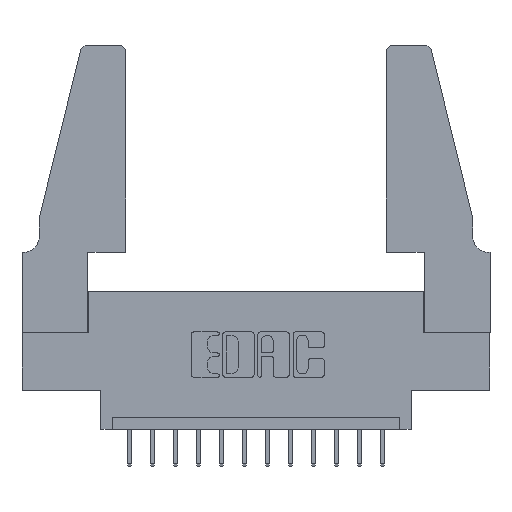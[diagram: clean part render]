
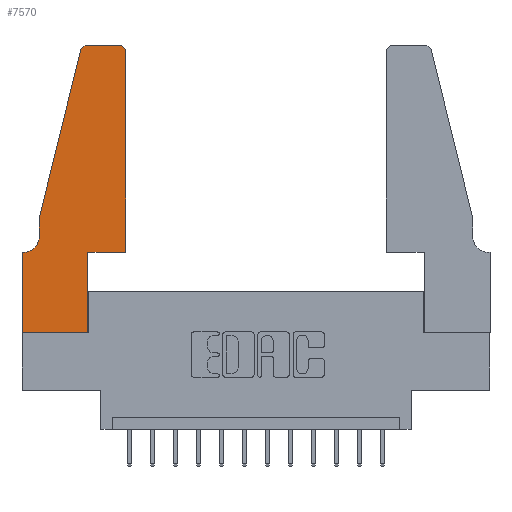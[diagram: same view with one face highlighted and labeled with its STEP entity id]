
A CAD part, top view. The second image highlights one B-rep face of the part: STEP entity #7570.
In plain terms, the highlighted planar face has unit normal (0, 0, 1).
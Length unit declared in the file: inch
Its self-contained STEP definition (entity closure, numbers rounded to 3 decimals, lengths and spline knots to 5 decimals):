
#68 = DIRECTION ( 'NONE',  ( 1., 0., 0. ) ) ;
#298 = CARTESIAN_POINT ( 'NONE',  ( 0.284, 1.22, 0.37 ) ) ;
#431 = VECTOR ( 'NONE', #9985, 39.37008 ) ;
#708 = EDGE_CURVE ( 'NONE', #6608, #3818, #10420, .T. ) ;
#802 = CIRCLE ( 'NONE', #4321, 0.03 ) ;
#808 = ORIENTED_EDGE ( 'NONE', *, *, #11677, .T. ) ;
#884 = DIRECTION ( 'NONE',  ( 0., 0., -1. ) ) ;
#943 = ORIENTED_EDGE ( 'NONE', *, *, #7886, .T. ) ;
#946 = CARTESIAN_POINT ( 'NONE',  ( 0.0755, 0.5, 0.37 ) ) ;
#1165 = ORIENTED_EDGE ( 'NONE', *, *, #3841, .T. ) ;
#1314 = CARTESIAN_POINT ( 'NONE',  ( 0.4205, 1.22, 0.37 ) ) ;
#1512 = DIRECTION ( 'NONE',  ( 0., 0., 1. ) ) ;
#1596 = CARTESIAN_POINT ( 'NONE',  ( 0., 0., 0.37 ) ) ;
#1765 = DIRECTION ( 'NONE',  ( -1., 0., 0. ) ) ;
#1864 = CARTESIAN_POINT ( 'NONE',  ( 0.4505, 1.22, 0.37 ) ) ;
#1882 = AXIS2_PLACEMENT_3D ( 'NONE', #9952, #1512, #10059 ) ;
#1934 = CARTESIAN_POINT ( 'NONE',  ( 0.0055, 0.35, 0.37 ) ) ;
#2064 = ORIENTED_EDGE ( 'NONE', *, *, #13709, .T. ) ;
#2082 = DIRECTION ( 'NONE',  ( -1., 0., 0. ) ) ;
#2103 = LINE ( 'NONE', #9622, #11247 ) ;
#2269 = CARTESIAN_POINT ( 'NONE',  ( 0.0755, 0.5, 0.37 ) ) ;
#2317 = DIRECTION ( 'NONE',  ( 0., 1., 0. ) ) ;
#2415 = DIRECTION ( 'NONE',  ( 0., 0., 1. ) ) ;
#2474 = AXIS2_PLACEMENT_3D ( 'NONE', #298, #5638, #11033 ) ;
#2614 = VERTEX_POINT ( 'NONE', #946 ) ;
#2679 = DIRECTION ( 'NONE',  ( 0., 1., 0. ) ) ;
#2787 = ORIENTED_EDGE ( 'NONE', *, *, #708, .T. ) ;
#2917 = VERTEX_POINT ( 'NONE', #4544 ) ;
#2943 = VECTOR ( 'NONE', #2679, 39.37008 ) ;
#3301 = VECTOR ( 'NONE', #11017, 39.37008 ) ;
#3420 = VECTOR ( 'NONE', #1765, 39.37008 ) ;
#3619 = EDGE_CURVE ( 'NONE', #13952, #6608, #2103, .T. ) ;
#3759 = CIRCLE ( 'NONE', #2474, 0.03 ) ;
#3818 = VERTEX_POINT ( 'NONE', #1864 ) ;
#3841 = EDGE_CURVE ( 'NONE', #4754, #2917, #9723, .T. ) ;
#4100 = CARTESIAN_POINT ( 'NONE',  ( 0.2605, 1.25, 0.37 ) ) ;
#4321 = AXIS2_PLACEMENT_3D ( 'NONE', #1314, #2415, #10714 ) ;
#4325 = VECTOR ( 'NONE', #10924, 39.37008 ) ;
#4544 = CARTESIAN_POINT ( 'NONE',  ( 0., 0.35, 0.37 ) ) ;
#4637 = CARTESIAN_POINT ( 'NONE',  ( 0., 0., 0.37 ) ) ;
#4721 = CARTESIAN_POINT ( 'NONE',  ( 0.2865, 0.35, 0.37 ) ) ;
#4754 = VERTEX_POINT ( 'NONE', #1934 ) ;
#4824 = VERTEX_POINT ( 'NONE', #4637 ) ;
#4888 = FACE_OUTER_BOUND ( 'NONE', #7447, .T. ) ;
#4907 = LINE ( 'NONE', #4100, #431 ) ;
#5067 = CARTESIAN_POINT ( 'NONE',  ( 0.0755, 0.5, 0.37 ) ) ;
#5089 = LINE ( 'NONE', #7706, #9004 ) ;
#5638 = DIRECTION ( 'NONE',  ( 0., 0., 1. ) ) ;
#5886 = EDGE_CURVE ( 'NONE', #12914, #4754, #10358, .T. ) ;
#6024 = VERTEX_POINT ( 'NONE', #11840 ) ;
#6356 = LINE ( 'NONE', #5067, #4325 ) ;
#6435 = DIRECTION ( 'NONE',  ( 0., -1., 0. ) ) ;
#6548 = CARTESIAN_POINT ( 'NONE',  ( 0.0755, 0.35, 0.37 ) ) ;
#6608 = VERTEX_POINT ( 'NONE', #14687 ) ;
#6820 = LINE ( 'NONE', #2269, #3301 ) ;
#7304 = ORIENTED_EDGE ( 'NONE', *, *, #13978, .T. ) ;
#7447 = EDGE_LOOP ( 'NONE', ( #10172, #943, #808, #7800, #12743, #1165, #2064, #10855, #14160, #7622, #2787, #7304 ) ) ;
#7570 = ADVANCED_FACE ( 'NONE', ( #4888 ), #9792, .T. ) ;
#7611 = CARTESIAN_POINT ( 'NONE',  ( 0.284, 1.25, 0.37 ) ) ;
#7622 = ORIENTED_EDGE ( 'NONE', *, *, #3619, .T. ) ;
#7673 = LINE ( 'NONE', #1596, #11987 ) ;
#7706 = CARTESIAN_POINT ( 'NONE',  ( 0.2865, 0.35, 0.37 ) ) ;
#7800 = ORIENTED_EDGE ( 'NONE', *, *, #14183, .T. ) ;
#7886 = EDGE_CURVE ( 'NONE', #14232, #12232, #3759, .T. ) ;
#8190 = CARTESIAN_POINT ( 'NONE',  ( 0.25487, 1.22718, 0.37 ) ) ;
#9004 = VECTOR ( 'NONE', #2317, 39.37008 ) ;
#9622 = CARTESIAN_POINT ( 'NONE',  ( 0.4505, 0.35, 0.37 ) ) ;
#9723 = LINE ( 'NONE', #6548, #3420 ) ;
#9792 = PLANE ( 'NONE',  #1882 ) ;
#9952 = CARTESIAN_POINT ( 'NONE',  ( 0., 0.35, 0.37 ) ) ;
#9985 = DIRECTION ( 'NONE',  ( -1., 0., 0. ) ) ;
#10057 = CARTESIAN_POINT ( 'NONE',  ( 0.0755, 0.42, 0.37 ) ) ;
#10059 = DIRECTION ( 'NONE',  ( 1., 0., 0. ) ) ;
#10172 = ORIENTED_EDGE ( 'NONE', *, *, #13643, .T. ) ;
#10358 = CIRCLE ( 'NONE', #13635, 0.07 ) ;
#10420 = LINE ( 'NONE', #13392, #2943 ) ;
#10455 = LINE ( 'NONE', #13163, #14366 ) ;
#10714 = DIRECTION ( 'NONE',  ( 1., 0., 0. ) ) ;
#10855 = ORIENTED_EDGE ( 'NONE', *, *, #15057, .T. ) ;
#10924 = DIRECTION ( 'NONE',  ( 0., -1., 0. ) ) ;
#11017 = DIRECTION ( 'NONE',  ( -0.239, -0.971, 0. ) ) ;
#11033 = DIRECTION ( 'NONE',  ( 1., 0., 0. ) ) ;
#11247 = VECTOR ( 'NONE', #14390, 39.37008 ) ;
#11677 = EDGE_CURVE ( 'NONE', #12232, #2614, #6820, .T. ) ;
#11840 = CARTESIAN_POINT ( 'NONE',  ( 0.2865, 0., 0.37 ) ) ;
#11987 = VECTOR ( 'NONE', #6435, 39.37008 ) ;
#12030 = CARTESIAN_POINT ( 'NONE',  ( 0.4205, 1.25, 0.37 ) ) ;
#12232 = VERTEX_POINT ( 'NONE', #8190 ) ;
#12540 = EDGE_CURVE ( 'NONE', #6024, #13952, #5089, .T. ) ;
#12743 = ORIENTED_EDGE ( 'NONE', *, *, #5886, .T. ) ;
#12914 = VERTEX_POINT ( 'NONE', #10057 ) ;
#13019 = VERTEX_POINT ( 'NONE', #12030 ) ;
#13163 = CARTESIAN_POINT ( 'NONE',  ( 0., 0., 0.37 ) ) ;
#13392 = CARTESIAN_POINT ( 'NONE',  ( 0.4505, 0.35, 0.37 ) ) ;
#13635 = AXIS2_PLACEMENT_3D ( 'NONE', #15314, #884, #2082 ) ;
#13643 = EDGE_CURVE ( 'NONE', #13019, #14232, #4907, .T. ) ;
#13709 = EDGE_CURVE ( 'NONE', #2917, #4824, #7673, .T. ) ;
#13952 = VERTEX_POINT ( 'NONE', #4721 ) ;
#13978 = EDGE_CURVE ( 'NONE', #3818, #13019, #802, .T. ) ;
#14160 = ORIENTED_EDGE ( 'NONE', *, *, #12540, .T. ) ;
#14183 = EDGE_CURVE ( 'NONE', #2614, #12914, #6356, .T. ) ;
#14232 = VERTEX_POINT ( 'NONE', #7611 ) ;
#14366 = VECTOR ( 'NONE', #68, 39.37008 ) ;
#14390 = DIRECTION ( 'NONE',  ( 1., 0., 0. ) ) ;
#14687 = CARTESIAN_POINT ( 'NONE',  ( 0.4505, 0.35, 0.37 ) ) ;
#15057 = EDGE_CURVE ( 'NONE', #4824, #6024, #10455, .T. ) ;
#15314 = CARTESIAN_POINT ( 'NONE',  ( 0.0055, 0.42, 0.37 ) ) ;
